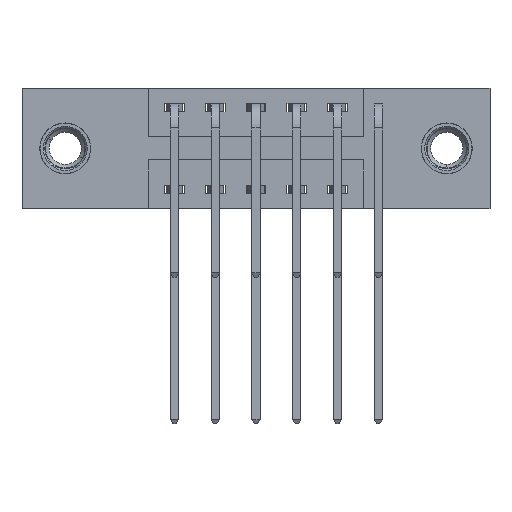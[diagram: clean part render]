
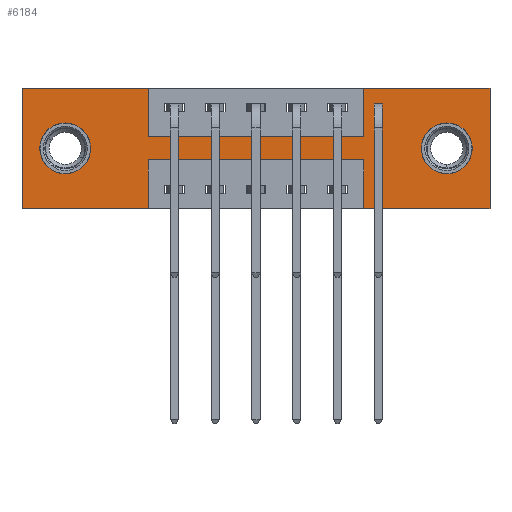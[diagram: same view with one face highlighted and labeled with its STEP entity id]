
A CAD part, front view. The second image highlights one B-rep face of the part: STEP entity #6184.
In plain terms, the highlighted planar face has unit normal (0, -1, 0).
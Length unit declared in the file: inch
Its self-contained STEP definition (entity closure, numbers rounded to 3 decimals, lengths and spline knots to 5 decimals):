
#91 = EDGE_CURVE ( 'NONE', #5293, #3443, #2855, .T. ) ;
#193 = DIRECTION ( 'NONE',  ( 0., 0., 1. ) ) ;
#387 = ORIENTED_EDGE ( 'NONE', *, *, #1471, .F. ) ;
#395 = CARTESIAN_POINT ( 'NONE',  ( 0., 0., 0. ) ) ;
#423 = VERTEX_POINT ( 'NONE', #5628 ) ;
#426 = LINE ( 'NONE', #3076, #10443 ) ;
#430 = LINE ( 'NONE', #1623, #4614 ) ;
#439 = CARTESIAN_POINT ( 'NONE',  ( 0.3875, 0., -0.15 ) ) ;
#474 = AXIS2_PLACEMENT_3D ( 'NONE', #3174, #10805, #8275 ) ;
#576 = CARTESIAN_POINT ( 'NONE',  ( 1.3025, 0., -0.263 ) ) ;
#595 = FACE_BOUND ( 'NONE', #2580, .T. ) ;
#790 = EDGE_CURVE ( 'NONE', #8055, #6637, #10884, .T. ) ;
#836 = AXIS2_PLACEMENT_3D ( 'NONE', #1685, #5184, #9255 ) ;
#852 = CARTESIAN_POINT ( 'NONE',  ( 0.1325, 0., -0.263 ) ) ;
#1037 = ORIENTED_EDGE ( 'NONE', *, *, #790, .T. ) ;
#1180 = VECTOR ( 'NONE', #7426, 39.37008 ) ;
#1192 = DIRECTION ( 'NONE',  ( 0., 0., -1. ) ) ;
#1245 = CARTESIAN_POINT ( 'NONE',  ( 1.435, 0., 0. ) ) ;
#1270 = ORIENTED_EDGE ( 'NONE', *, *, #2819, .F. ) ;
#1375 = DIRECTION ( 'NONE',  ( 1., 0., 0. ) ) ;
#1471 = EDGE_CURVE ( 'NONE', #7982, #4016, #6565, .T. ) ;
#1476 = LINE ( 'NONE', #2935, #8614 ) ;
#1541 = CARTESIAN_POINT ( 'NONE',  ( 1.0475, 0., -0.22 ) ) ;
#1582 = FACE_BOUND ( 'NONE', #8165, .T. ) ;
#1589 = EDGE_CURVE ( 'NONE', #2635, #7982, #3369, .T. ) ;
#1623 = CARTESIAN_POINT ( 'NONE',  ( 1.0475, 0., -0.37 ) ) ;
#1685 = CARTESIAN_POINT ( 'NONE',  ( 1.3025, 0., -0.185 ) ) ;
#1734 = ORIENTED_EDGE ( 'NONE', *, *, #3660, .F. ) ;
#1891 = VECTOR ( 'NONE', #2826, 39.37008 ) ;
#1901 = VECTOR ( 'NONE', #1192, 39.37008 ) ;
#1938 = AXIS2_PLACEMENT_3D ( 'NONE', #11118, #5083, #6617 ) ;
#2087 = VERTEX_POINT ( 'NONE', #6238 ) ;
#2120 = ORIENTED_EDGE ( 'NONE', *, *, #6257, .F. ) ;
#2178 = VERTEX_POINT ( 'NONE', #7721 ) ;
#2243 = EDGE_LOOP ( 'NONE', ( #10639, #6568, #10611, #7109, #1270, #8059, #2120, #387, #10142, #1734, #10726, #7032 ) ) ;
#2255 = LINE ( 'NONE', #395, #9199 ) ;
#2290 = CARTESIAN_POINT ( 'NONE',  ( 0.3875, 0., -0.15 ) ) ;
#2363 = CARTESIAN_POINT ( 'NONE',  ( 0.3875, 0., 0. ) ) ;
#2378 = DIRECTION ( 'NONE',  ( 0., 0., 1. ) ) ;
#2436 = CIRCLE ( 'NONE', #6812, 0.078 ) ;
#2523 = CARTESIAN_POINT ( 'NONE',  ( 1.3025, 0., -0.185 ) ) ;
#2580 = EDGE_LOOP ( 'NONE', ( #3834, #1037 ) ) ;
#2635 = VERTEX_POINT ( 'NONE', #2363 ) ;
#2819 = EDGE_CURVE ( 'NONE', #3509, #4646, #4903, .T. ) ;
#2826 = DIRECTION ( 'NONE',  ( -1., 0., 0. ) ) ;
#2855 = CIRCLE ( 'NONE', #836, 0.078 ) ;
#2917 = CARTESIAN_POINT ( 'NONE',  ( 0.3875, 0., -0.37 ) ) ;
#2935 = CARTESIAN_POINT ( 'NONE',  ( 0.3875, 0., -0.22 ) ) ;
#3076 = CARTESIAN_POINT ( 'NONE',  ( 0., 0., 0. ) ) ;
#3174 = CARTESIAN_POINT ( 'NONE',  ( 0.1325, 0., -0.185 ) ) ;
#3196 = VECTOR ( 'NONE', #9141, 39.37008 ) ;
#3253 = LINE ( 'NONE', #4088, #3196 ) ;
#3369 = LINE ( 'NONE', #6843, #11001 ) ;
#3443 = VERTEX_POINT ( 'NONE', #576 ) ;
#3509 = VERTEX_POINT ( 'NONE', #10410 ) ;
#3660 = EDGE_CURVE ( 'NONE', #2087, #2635, #2255, .T. ) ;
#3664 = CARTESIAN_POINT ( 'NONE',  ( 0., 0., 0. ) ) ;
#3834 = ORIENTED_EDGE ( 'NONE', *, *, #6070, .T. ) ;
#3986 = DIRECTION ( 'NONE',  ( 0., 0., 1. ) ) ;
#4016 = VERTEX_POINT ( 'NONE', #6920 ) ;
#4088 = CARTESIAN_POINT ( 'NONE',  ( 0., 0., -0.37 ) ) ;
#4144 = ORIENTED_EDGE ( 'NONE', *, *, #11025, .T. ) ;
#4614 = VECTOR ( 'NONE', #2378, 39.37008 ) ;
#4646 = VERTEX_POINT ( 'NONE', #5471 ) ;
#4749 = EDGE_CURVE ( 'NONE', #423, #10909, #430, .T. ) ;
#4903 = LINE ( 'NONE', #1245, #1901 ) ;
#4905 = FACE_OUTER_BOUND ( 'NONE', #2243, .T. ) ;
#5083 = DIRECTION ( 'NONE',  ( 0., -1., 0. ) ) ;
#5184 = DIRECTION ( 'NONE',  ( 0., 1., 0. ) ) ;
#5293 = VERTEX_POINT ( 'NONE', #7039 ) ;
#5300 = EDGE_CURVE ( 'NONE', #6403, #2087, #8769, .T. ) ;
#5471 = CARTESIAN_POINT ( 'NONE',  ( 1.435, 0., -0.37 ) ) ;
#5509 = EDGE_CURVE ( 'NONE', #2178, #9067, #10685, .T. ) ;
#5628 = CARTESIAN_POINT ( 'NONE',  ( 1.0475, 0., -0.37 ) ) ;
#5999 = DIRECTION ( 'NONE',  ( 0., 1., 0. ) ) ;
#6070 = EDGE_CURVE ( 'NONE', #6637, #8055, #2436, .T. ) ;
#6184 = ADVANCED_FACE ( 'NONE', ( #1582, #595, #4905 ), #10254, .T. ) ;
#6238 = CARTESIAN_POINT ( 'NONE',  ( 0., 0., 0. ) ) ;
#6257 = EDGE_CURVE ( 'NONE', #4016, #9624, #6735, .T. ) ;
#6403 = VERTEX_POINT ( 'NONE', #8689 ) ;
#6565 = LINE ( 'NONE', #2290, #7885 ) ;
#6568 = ORIENTED_EDGE ( 'NONE', *, *, #10370, .F. ) ;
#6617 = DIRECTION ( 'NONE',  ( 0., 0., -1. ) ) ;
#6637 = VERTEX_POINT ( 'NONE', #7336 ) ;
#6699 = EDGE_CURVE ( 'NONE', #4646, #423, #3253, .T. ) ;
#6735 = LINE ( 'NONE', #9261, #9564 ) ;
#6812 = AXIS2_PLACEMENT_3D ( 'NONE', #8016, #10723, #193 ) ;
#6843 = CARTESIAN_POINT ( 'NONE',  ( 0.3875, 0., 0. ) ) ;
#6920 = CARTESIAN_POINT ( 'NONE',  ( 1.0475, 0., -0.15 ) ) ;
#7032 = ORIENTED_EDGE ( 'NONE', *, *, #10257, .F. ) ;
#7039 = CARTESIAN_POINT ( 'NONE',  ( 1.3025, 0., -0.107 ) ) ;
#7109 = ORIENTED_EDGE ( 'NONE', *, *, #6699, .F. ) ;
#7149 = LINE ( 'NONE', #9650, #1891 ) ;
#7336 = CARTESIAN_POINT ( 'NONE',  ( 0.1325, 0., -0.107 ) ) ;
#7426 = DIRECTION ( 'NONE',  ( 0., 0., -1. ) ) ;
#7512 = DIRECTION ( 'NONE',  ( 1., 0., 0. ) ) ;
#7721 = CARTESIAN_POINT ( 'NONE',  ( 0.3875, 0., -0.22 ) ) ;
#7729 = VECTOR ( 'NONE', #8026, 39.37008 ) ;
#7732 = AXIS2_PLACEMENT_3D ( 'NONE', #2523, #5999, #9451 ) ;
#7885 = VECTOR ( 'NONE', #1375, 39.37008 ) ;
#7982 = VERTEX_POINT ( 'NONE', #439 ) ;
#8016 = CARTESIAN_POINT ( 'NONE',  ( 0.1325, 0., -0.185 ) ) ;
#8026 = DIRECTION ( 'NONE',  ( 0., 0., 1. ) ) ;
#8055 = VERTEX_POINT ( 'NONE', #852 ) ;
#8059 = ORIENTED_EDGE ( 'NONE', *, *, #9647, .F. ) ;
#8146 = CARTESIAN_POINT ( 'NONE',  ( 0.3875, 0., -0.37 ) ) ;
#8165 = EDGE_LOOP ( 'NONE', ( #11125, #4144 ) ) ;
#8275 = DIRECTION ( 'NONE',  ( 0., 0., 1. ) ) ;
#8614 = VECTOR ( 'NONE', #10866, 39.37008 ) ;
#8689 = CARTESIAN_POINT ( 'NONE',  ( 0., 0., -0.37 ) ) ;
#8769 = LINE ( 'NONE', #3664, #7729 ) ;
#8891 = DIRECTION ( 'NONE',  ( 0., 0., -1. ) ) ;
#8982 = CARTESIAN_POINT ( 'NONE',  ( 1.0475, 0., 0. ) ) ;
#9067 = VERTEX_POINT ( 'NONE', #2917 ) ;
#9141 = DIRECTION ( 'NONE',  ( -1., 0., 0. ) ) ;
#9174 = CIRCLE ( 'NONE', #7732, 0.078 ) ;
#9199 = VECTOR ( 'NONE', #10000, 39.37008 ) ;
#9255 = DIRECTION ( 'NONE',  ( 0., 0., -1. ) ) ;
#9261 = CARTESIAN_POINT ( 'NONE',  ( 1.0475, 0., 0. ) ) ;
#9451 = DIRECTION ( 'NONE',  ( 0., 0., -1. ) ) ;
#9564 = VECTOR ( 'NONE', #3986, 39.37008 ) ;
#9624 = VERTEX_POINT ( 'NONE', #8982 ) ;
#9647 = EDGE_CURVE ( 'NONE', #9624, #3509, #426, .T. ) ;
#9650 = CARTESIAN_POINT ( 'NONE',  ( 0., 0., -0.37 ) ) ;
#10000 = DIRECTION ( 'NONE',  ( 1., 0., 0. ) ) ;
#10142 = ORIENTED_EDGE ( 'NONE', *, *, #1589, .F. ) ;
#10254 = PLANE ( 'NONE',  #1938 ) ;
#10257 = EDGE_CURVE ( 'NONE', #9067, #6403, #7149, .T. ) ;
#10370 = EDGE_CURVE ( 'NONE', #10909, #2178, #1476, .T. ) ;
#10410 = CARTESIAN_POINT ( 'NONE',  ( 1.435, 0., 0. ) ) ;
#10443 = VECTOR ( 'NONE', #7512, 39.37008 ) ;
#10611 = ORIENTED_EDGE ( 'NONE', *, *, #4749, .F. ) ;
#10639 = ORIENTED_EDGE ( 'NONE', *, *, #5509, .F. ) ;
#10685 = LINE ( 'NONE', #8146, #1180 ) ;
#10723 = DIRECTION ( 'NONE',  ( 0., 1., 0. ) ) ;
#10726 = ORIENTED_EDGE ( 'NONE', *, *, #5300, .F. ) ;
#10805 = DIRECTION ( 'NONE',  ( 0., 1., 0. ) ) ;
#10866 = DIRECTION ( 'NONE',  ( -1., 0., 0. ) ) ;
#10884 = CIRCLE ( 'NONE', #474, 0.078 ) ;
#10909 = VERTEX_POINT ( 'NONE', #1541 ) ;
#11001 = VECTOR ( 'NONE', #8891, 39.37008 ) ;
#11025 = EDGE_CURVE ( 'NONE', #3443, #5293, #9174, .T. ) ;
#11118 = CARTESIAN_POINT ( 'NONE',  ( 0., 0., -0.37 ) ) ;
#11125 = ORIENTED_EDGE ( 'NONE', *, *, #91, .T. ) ;
